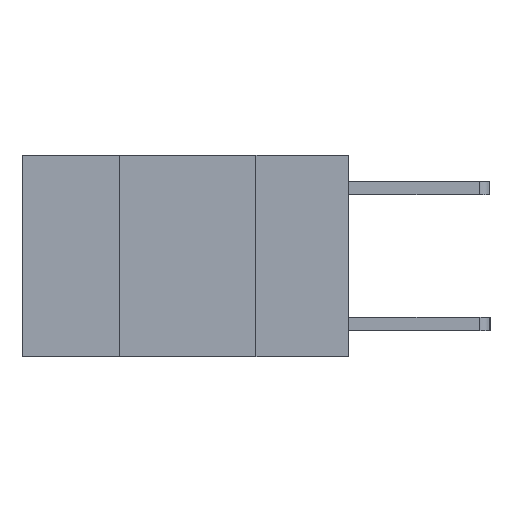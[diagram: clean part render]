
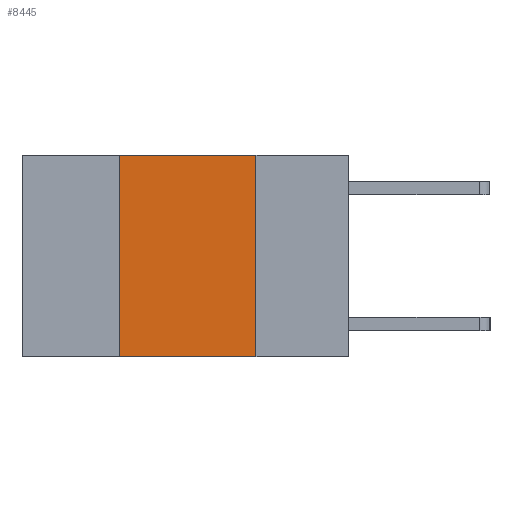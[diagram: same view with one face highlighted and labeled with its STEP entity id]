
A CAD part, left-side view. The second image highlights one B-rep face of the part: STEP entity #8445.
In plain terms, the highlighted planar face has unit normal (-1, 0, 0).
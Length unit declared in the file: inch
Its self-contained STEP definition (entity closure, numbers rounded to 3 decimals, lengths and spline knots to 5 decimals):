
#100 = LINE ( 'NONE', #852, #3494 ) ;
#450 = VERTEX_POINT ( 'NONE', #3564 ) ;
#490 = ORIENTED_EDGE ( 'NONE', *, *, #906, .F. ) ;
#643 = CARTESIAN_POINT ( 'NONE',  ( 0., 0.42, -0.37 ) ) ;
#650 = LINE ( 'NONE', #2547, #5745 ) ;
#704 = ORIENTED_EDGE ( 'NONE', *, *, #7042, .F. ) ;
#852 = CARTESIAN_POINT ( 'NONE',  ( 0., 0.42, 0. ) ) ;
#906 = EDGE_CURVE ( 'NONE', #8033, #450, #650, .T. ) ;
#908 = ORIENTED_EDGE ( 'NONE', *, *, #6836, .T. ) ;
#1343 = DIRECTION ( 'NONE',  ( 0., -1., 0. ) ) ;
#2547 = CARTESIAN_POINT ( 'NONE',  ( 0., 0.6, 0. ) ) ;
#2774 = LINE ( 'NONE', #7329, #6087 ) ;
#3131 = PLANE ( 'NONE',  #5952 ) ;
#3494 = VECTOR ( 'NONE', #4856, 39.37008 ) ;
#3520 = FACE_OUTER_BOUND ( 'NONE', #4636, .T. ) ;
#3564 = CARTESIAN_POINT ( 'NONE',  ( 0., 0.17, 0. ) ) ;
#3794 = DIRECTION ( 'NONE',  ( 1., 0., 0. ) ) ;
#4011 = CARTESIAN_POINT ( 'NONE',  ( 0., 0.6, -0.37 ) ) ;
#4255 = DIRECTION ( 'NONE',  ( 0., -1., 0. ) ) ;
#4545 = EDGE_CURVE ( 'NONE', #450, #8336, #2774, .T. ) ;
#4636 = EDGE_LOOP ( 'NONE', ( #4747, #490, #704, #908 ) ) ;
#4747 = ORIENTED_EDGE ( 'NONE', *, *, #4545, .F. ) ;
#4856 = DIRECTION ( 'NONE',  ( 0., 0., 1. ) ) ;
#5745 = VECTOR ( 'NONE', #4255, 39.37008 ) ;
#5952 = AXIS2_PLACEMENT_3D ( 'NONE', #7781, #3794, #8447 ) ;
#6087 = VECTOR ( 'NONE', #7909, 39.37008 ) ;
#6692 = VECTOR ( 'NONE', #1343, 39.37008 ) ;
#6836 = EDGE_CURVE ( 'NONE', #7489, #8336, #8476, .T. ) ;
#6986 = CARTESIAN_POINT ( 'NONE',  ( 0., 0.17, -0.37 ) ) ;
#7042 = EDGE_CURVE ( 'NONE', #7489, #8033, #100, .T. ) ;
#7329 = CARTESIAN_POINT ( 'NONE',  ( 0., 0.17, 0. ) ) ;
#7489 = VERTEX_POINT ( 'NONE', #643 ) ;
#7781 = CARTESIAN_POINT ( 'NONE',  ( 0., 0.6, 0. ) ) ;
#7909 = DIRECTION ( 'NONE',  ( 0., 0., -1. ) ) ;
#8033 = VERTEX_POINT ( 'NONE', #8567 ) ;
#8336 = VERTEX_POINT ( 'NONE', #6986 ) ;
#8445 = ADVANCED_FACE ( 'NONE', ( #3520 ), #3131, .F. ) ;
#8447 = DIRECTION ( 'NONE',  ( 0., 0., -1. ) ) ;
#8476 = LINE ( 'NONE', #4011, #6692 ) ;
#8567 = CARTESIAN_POINT ( 'NONE',  ( 0., 0.42, 0. ) ) ;
